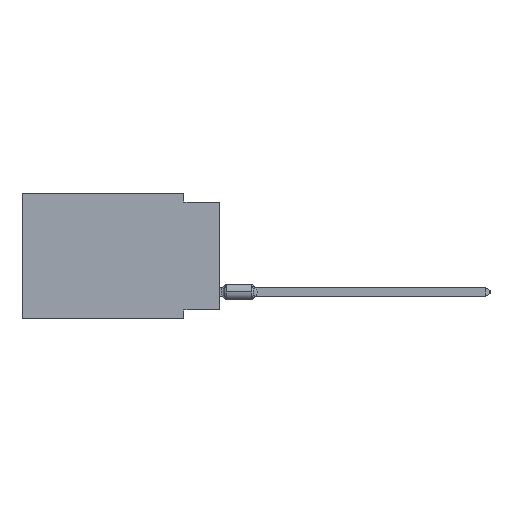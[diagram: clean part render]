
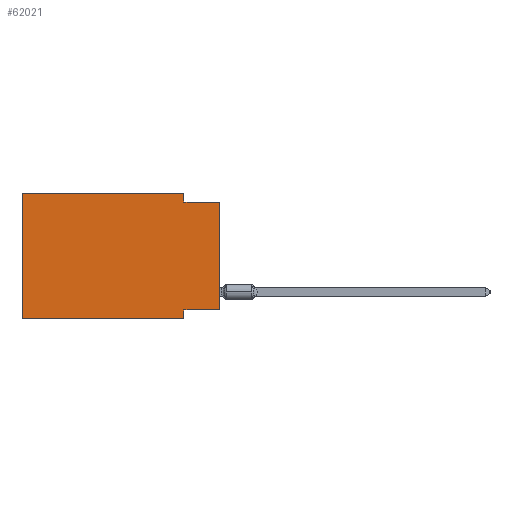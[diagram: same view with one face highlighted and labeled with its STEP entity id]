
A CAD part, left-side view. The second image highlights one B-rep face of the part: STEP entity #62021.
In plain terms, the highlighted planar face has unit normal (-1, 0, 0).
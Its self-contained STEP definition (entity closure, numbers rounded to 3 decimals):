
#558 = DIRECTION ( 'NONE',  ( 0., -1., 0. ) ) ;
#2617 = CARTESIAN_POINT ( 'NONE',  ( 0., 2.54, -8.89 ) ) ;
#2979 = CARTESIAN_POINT ( 'NONE',  ( 0., 2.54, 0. ) ) ;
#3681 = LINE ( 'NONE', #11577, #29238 ) ;
#5842 = LINE ( 'NONE', #47271, #10572 ) ;
#8000 = LINE ( 'NONE', #14980, #32094 ) ;
#8103 = EDGE_CURVE ( 'NONE', #67742, #67989, #8000, .T. ) ;
#9367 = EDGE_CURVE ( 'NONE', #58755, #85313, #60865, .T. ) ;
#10572 = VECTOR ( 'NONE', #68222, 1000. ) ;
#11069 = CARTESIAN_POINT ( 'NONE',  ( 0., 13.97, -8.89 ) ) ;
#11160 = LINE ( 'NONE', #39539, #67023 ) ;
#11577 = CARTESIAN_POINT ( 'NONE',  ( 0., 13.97, 0. ) ) ;
#13242 = EDGE_CURVE ( 'NONE', #27895, #40255, #16676, .T. ) ;
#14980 = CARTESIAN_POINT ( 'NONE',  ( 0., 13.97, 0. ) ) ;
#15363 = ORIENTED_EDGE ( 'NONE', *, *, #43617, .F. ) ;
#15602 = FACE_OUTER_BOUND ( 'NONE', #62035, .T. ) ;
#16676 = LINE ( 'NONE', #11069, #26555 ) ;
#18228 = EDGE_CURVE ( 'NONE', #27189, #40255, #24697, .T. ) ;
#21766 = VECTOR ( 'NONE', #31827, 1000. ) ;
#23476 = LINE ( 'NONE', #2979, #21766 ) ;
#24697 = LINE ( 'NONE', #46116, #61237 ) ;
#26133 = CARTESIAN_POINT ( 'NONE',  ( 0., 13.97, -8.89 ) ) ;
#26555 = VECTOR ( 'NONE', #74820, 1000. ) ;
#27189 = VERTEX_POINT ( 'NONE', #62305 ) ;
#27895 = VERTEX_POINT ( 'NONE', #26133 ) ;
#29238 = VECTOR ( 'NONE', #46042, 1000. ) ;
#29962 = ORIENTED_EDGE ( 'NONE', *, *, #8103, .F. ) ;
#31827 = DIRECTION ( 'NONE',  ( 0., 0., -1. ) ) ;
#32040 = EDGE_CURVE ( 'NONE', #36393, #85313, #11160, .T. ) ;
#32094 = VECTOR ( 'NONE', #558, 1000. ) ;
#33078 = CARTESIAN_POINT ( 'NONE',  ( 0., 2.54, -0.635 ) ) ;
#33250 = ORIENTED_EDGE ( 'NONE', *, *, #9367, .T. ) ;
#35655 = DIRECTION ( 'NONE',  ( 0., -1., 0. ) ) ;
#36393 = VERTEX_POINT ( 'NONE', #33078 ) ;
#36778 = EDGE_CURVE ( 'NONE', #27895, #67742, #3681, .T. ) ;
#38072 = DIRECTION ( 'NONE',  ( 0., 0., 1. ) ) ;
#39539 = CARTESIAN_POINT ( 'NONE',  ( 0., 0., -0.635 ) ) ;
#39653 = ORIENTED_EDGE ( 'NONE', *, *, #32040, .F. ) ;
#40255 = VERTEX_POINT ( 'NONE', #2617 ) ;
#43617 = EDGE_CURVE ( 'NONE', #58755, #27189, #5842, .T. ) ;
#43705 = ORIENTED_EDGE ( 'NONE', *, *, #13242, .T. ) ;
#43989 = PLANE ( 'NONE',  #88504 ) ;
#46042 = DIRECTION ( 'NONE',  ( 0., 0., 1. ) ) ;
#46116 = CARTESIAN_POINT ( 'NONE',  ( 0., 2.54, -8.89 ) ) ;
#47271 = CARTESIAN_POINT ( 'NONE',  ( 0., 0., -8.255 ) ) ;
#48893 = ORIENTED_EDGE ( 'NONE', *, *, #18228, .F. ) ;
#55627 = EDGE_CURVE ( 'NONE', #67989, #36393, #23476, .T. ) ;
#58417 = DIRECTION ( 'NONE',  ( 1., 0., 0. ) ) ;
#58755 = VERTEX_POINT ( 'NONE', #64329 ) ;
#60081 = DIRECTION ( 'NONE',  ( 0., 0., -1. ) ) ;
#60865 = LINE ( 'NONE', #66008, #85737 ) ;
#60872 = CARTESIAN_POINT ( 'NONE',  ( 0., 0., -0.635 ) ) ;
#61237 = VECTOR ( 'NONE', #60081, 1000. ) ;
#62021 = ADVANCED_FACE ( 'NONE', ( #15602 ), #43989, .F. ) ;
#62035 = EDGE_LOOP ( 'NONE', ( #33250, #39653, #64161, #29962, #77066, #43705, #48893, #15363 ) ) ;
#62305 = CARTESIAN_POINT ( 'NONE',  ( 0., 2.54, -8.255 ) ) ;
#64161 = ORIENTED_EDGE ( 'NONE', *, *, #55627, .F. ) ;
#64329 = CARTESIAN_POINT ( 'NONE',  ( 0., 0., -8.255 ) ) ;
#65395 = CARTESIAN_POINT ( 'NONE',  ( 0., 13.97, 0. ) ) ;
#66008 = CARTESIAN_POINT ( 'NONE',  ( 0., 0., 0. ) ) ;
#67023 = VECTOR ( 'NONE', #35655, 1000. ) ;
#67742 = VERTEX_POINT ( 'NONE', #72467 ) ;
#67989 = VERTEX_POINT ( 'NONE', #70988 ) ;
#68222 = DIRECTION ( 'NONE',  ( 0., 1., 0. ) ) ;
#70988 = CARTESIAN_POINT ( 'NONE',  ( 0., 2.54, 0. ) ) ;
#72467 = CARTESIAN_POINT ( 'NONE',  ( 0., 13.97, 0. ) ) ;
#74820 = DIRECTION ( 'NONE',  ( 0., -1., 0. ) ) ;
#77066 = ORIENTED_EDGE ( 'NONE', *, *, #36778, .F. ) ;
#85313 = VERTEX_POINT ( 'NONE', #60872 ) ;
#85737 = VECTOR ( 'NONE', #38072, 1000. ) ;
#86806 = DIRECTION ( 'NONE',  ( 0., 0., -1. ) ) ;
#88504 = AXIS2_PLACEMENT_3D ( 'NONE', #65395, #58417, #86806 ) ;
